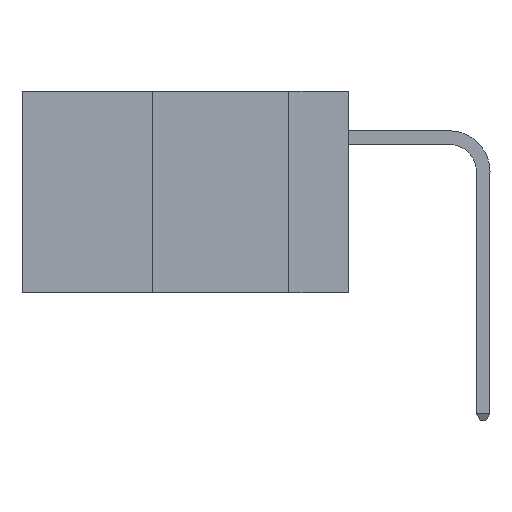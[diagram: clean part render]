
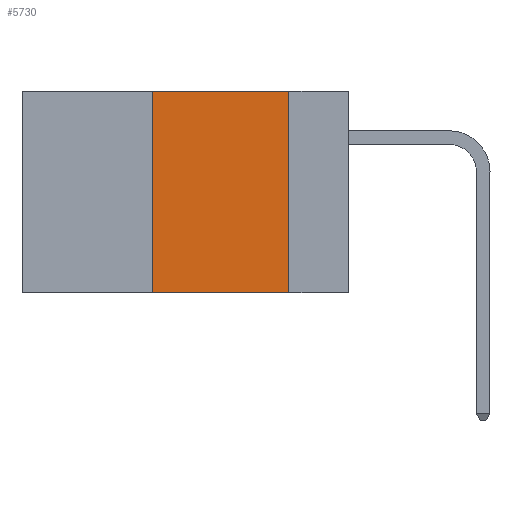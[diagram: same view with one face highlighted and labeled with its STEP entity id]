
A CAD part, left-side view. The second image highlights one B-rep face of the part: STEP entity #5730.
In plain terms, the highlighted planar face has unit normal (-1, 0, 0).
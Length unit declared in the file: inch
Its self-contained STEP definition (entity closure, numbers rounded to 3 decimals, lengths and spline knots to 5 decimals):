
#67 = EDGE_CURVE ( 'NONE', #15858, #19569, #17707, .T. ) ;
#1227 = LINE ( 'NONE', #14823, #4127 ) ;
#1532 = CARTESIAN_POINT ( 'NONE',  ( 0., 0.11, 0. ) ) ;
#1870 = FACE_OUTER_BOUND ( 'NONE', #14346, .T. ) ;
#2412 = DIRECTION ( 'NONE',  ( 0., 0., 1. ) ) ;
#3001 = CARTESIAN_POINT ( 'NONE',  ( 0., 0.36, 0. ) ) ;
#3612 = CARTESIAN_POINT ( 'NONE',  ( 0., 0.11, 0. ) ) ;
#3739 = PLANE ( 'NONE',  #6135 ) ;
#3852 = DIRECTION ( 'NONE',  ( 0., -1., 0. ) ) ;
#3874 = CARTESIAN_POINT ( 'NONE',  ( 0., 0.6, 0. ) ) ;
#4127 = VECTOR ( 'NONE', #2412, 39.37008 ) ;
#5104 = VERTEX_POINT ( 'NONE', #6172 ) ;
#5730 = ADVANCED_FACE ( 'NONE', ( #1870 ), #3739, .F. ) ;
#6135 = AXIS2_PLACEMENT_3D ( 'NONE', #3874, #16330, #10172 ) ;
#6172 = CARTESIAN_POINT ( 'NONE',  ( 0., 0.36, -0.37 ) ) ;
#6676 = ORIENTED_EDGE ( 'NONE', *, *, #67, .F. ) ;
#8068 = VECTOR ( 'NONE', #3852, 39.37008 ) ;
#8748 = CARTESIAN_POINT ( 'NONE',  ( 0., 0.11, -0.37 ) ) ;
#10172 = DIRECTION ( 'NONE',  ( 0., 0., -1. ) ) ;
#10595 = DIRECTION ( 'NONE',  ( 0., -1., 0. ) ) ;
#10620 = VERTEX_POINT ( 'NONE', #8748 ) ;
#10950 = VECTOR ( 'NONE', #10595, 39.37008 ) ;
#11321 = EDGE_CURVE ( 'NONE', #5104, #10620, #12206, .T. ) ;
#12206 = LINE ( 'NONE', #13116, #8068 ) ;
#13116 = CARTESIAN_POINT ( 'NONE',  ( 0., 0.6, -0.37 ) ) ;
#13693 = EDGE_CURVE ( 'NONE', #5104, #15858, #1227, .T. ) ;
#13709 = CARTESIAN_POINT ( 'NONE',  ( 0., 0.6, 0. ) ) ;
#13733 = ORIENTED_EDGE ( 'NONE', *, *, #13693, .F. ) ;
#14293 = LINE ( 'NONE', #1532, #17422 ) ;
#14346 = EDGE_LOOP ( 'NONE', ( #18082, #6676, #13733, #18333 ) ) ;
#14823 = CARTESIAN_POINT ( 'NONE',  ( 0., 0.36, 0. ) ) ;
#15858 = VERTEX_POINT ( 'NONE', #3001 ) ;
#16330 = DIRECTION ( 'NONE',  ( 1., 0., 0. ) ) ;
#17422 = VECTOR ( 'NONE', #20032, 39.37008 ) ;
#17707 = LINE ( 'NONE', #13709, #10950 ) ;
#18082 = ORIENTED_EDGE ( 'NONE', *, *, #18893, .F. ) ;
#18333 = ORIENTED_EDGE ( 'NONE', *, *, #11321, .T. ) ;
#18893 = EDGE_CURVE ( 'NONE', #19569, #10620, #14293, .T. ) ;
#19569 = VERTEX_POINT ( 'NONE', #3612 ) ;
#20032 = DIRECTION ( 'NONE',  ( 0., 0., -1. ) ) ;
